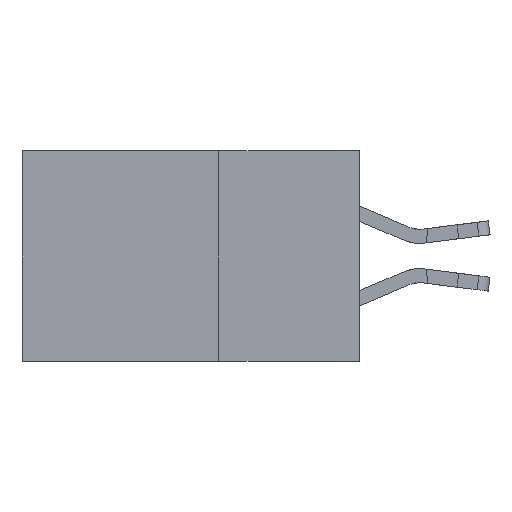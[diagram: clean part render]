
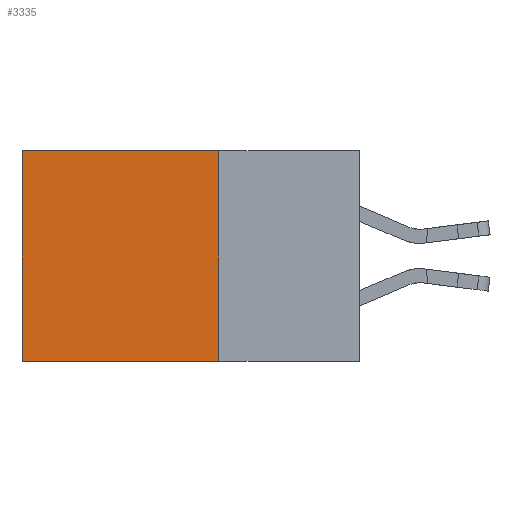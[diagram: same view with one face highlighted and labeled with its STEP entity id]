
A CAD part, left-side view. The second image highlights one B-rep face of the part: STEP entity #3335.
In plain terms, the highlighted planar face has unit normal (-1, 0, 0).
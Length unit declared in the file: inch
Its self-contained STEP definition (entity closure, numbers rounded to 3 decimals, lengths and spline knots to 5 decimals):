
#282 = VECTOR ( 'NONE', #4807, 39.37008 ) ;
#530 = EDGE_CURVE ( 'NONE', #6655, #5770, #13966, .T. ) ;
#631 = CARTESIAN_POINT ( 'NONE',  ( 0.2875, 0.6, -0.375 ) ) ;
#1252 = EDGE_LOOP ( 'NONE', ( #12183, #10328, #3078, #4360 ) ) ;
#1738 = CARTESIAN_POINT ( 'NONE',  ( 0.2875, 0.25, -0.375 ) ) ;
#2195 = CARTESIAN_POINT ( 'NONE',  ( 0.2875, 0.25, -0.375 ) ) ;
#2358 = PLANE ( 'NONE',  #12585 ) ;
#3078 = ORIENTED_EDGE ( 'NONE', *, *, #7748, .F. ) ;
#3269 = CARTESIAN_POINT ( 'NONE',  ( 0.2875, 0.6, -0.375 ) ) ;
#3335 = ADVANCED_FACE ( 'NONE', ( #3513 ), #2358, .F. ) ;
#3513 = FACE_OUTER_BOUND ( 'NONE', #1252, .T. ) ;
#3816 = DIRECTION ( 'NONE',  ( 0., 1., 0. ) ) ;
#4360 = ORIENTED_EDGE ( 'NONE', *, *, #8344, .T. ) ;
#4807 = DIRECTION ( 'NONE',  ( 0., 1., 0. ) ) ;
#4819 = DIRECTION ( 'NONE',  ( 1., 0., 0. ) ) ;
#5182 = VECTOR ( 'NONE', #3816, 39.37008 ) ;
#5192 = CARTESIAN_POINT ( 'NONE',  ( 0.2875, 0.25, -0.375 ) ) ;
#5289 = CARTESIAN_POINT ( 'NONE',  ( 0.2875, 0.6, 0. ) ) ;
#5770 = VERTEX_POINT ( 'NONE', #631 ) ;
#5988 = DIRECTION ( 'NONE',  ( 0., 0., -1. ) ) ;
#6628 = VERTEX_POINT ( 'NONE', #1738 ) ;
#6655 = VERTEX_POINT ( 'NONE', #5289 ) ;
#6905 = VECTOR ( 'NONE', #5988, 39.37008 ) ;
#7748 = EDGE_CURVE ( 'NONE', #11201, #6628, #9375, .T. ) ;
#7825 = DIRECTION ( 'NONE',  ( 0., 0., -1. ) ) ;
#8344 = EDGE_CURVE ( 'NONE', #11201, #6655, #12200, .T. ) ;
#9375 = LINE ( 'NONE', #10520, #6905 ) ;
#9519 = DIRECTION ( 'NONE',  ( 0., 0., -1. ) ) ;
#9544 = EDGE_CURVE ( 'NONE', #6628, #5770, #11043, .T. ) ;
#9833 = VECTOR ( 'NONE', #7825, 39.37008 ) ;
#10328 = ORIENTED_EDGE ( 'NONE', *, *, #9544, .F. ) ;
#10520 = CARTESIAN_POINT ( 'NONE',  ( 0.2875, 0.25, -0.375 ) ) ;
#10662 = CARTESIAN_POINT ( 'NONE',  ( 0.2875, 0.25, 0. ) ) ;
#11043 = LINE ( 'NONE', #5192, #5182 ) ;
#11201 = VERTEX_POINT ( 'NONE', #14354 ) ;
#12183 = ORIENTED_EDGE ( 'NONE', *, *, #530, .T. ) ;
#12200 = LINE ( 'NONE', #10662, #282 ) ;
#12585 = AXIS2_PLACEMENT_3D ( 'NONE', #2195, #4819, #9519 ) ;
#13966 = LINE ( 'NONE', #3269, #9833 ) ;
#14354 = CARTESIAN_POINT ( 'NONE',  ( 0.2875, 0.25, 0. ) ) ;
